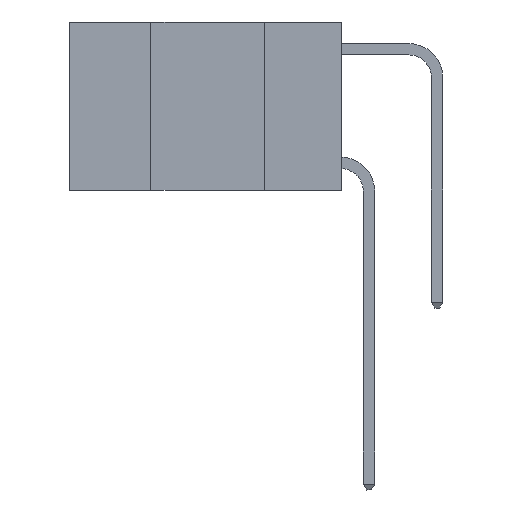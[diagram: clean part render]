
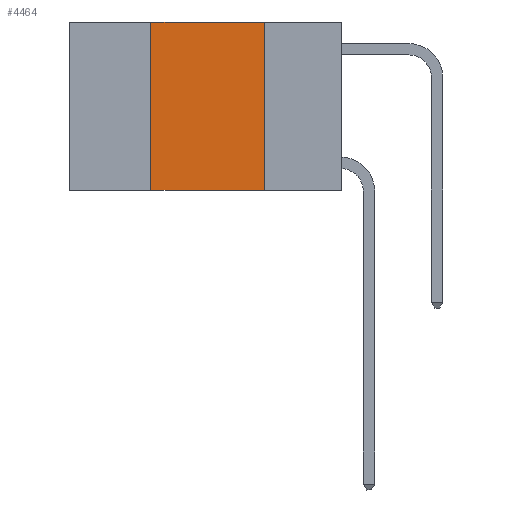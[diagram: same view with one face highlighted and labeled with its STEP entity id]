
A CAD part, left-side view. The second image highlights one B-rep face of the part: STEP entity #4464.
In plain terms, the highlighted planar face has unit normal (-1, 0, 0).
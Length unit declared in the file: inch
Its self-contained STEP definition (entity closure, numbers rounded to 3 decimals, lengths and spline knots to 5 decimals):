
#436 = DIRECTION ( 'NONE',  ( 0., 0., -1. ) ) ;
#487 = EDGE_CURVE ( 'NONE', #7042, #10571, #1868, .T. ) ;
#671 = CARTESIAN_POINT ( 'NONE',  ( 0., 0.6, 0. ) ) ;
#967 = LINE ( 'NONE', #9400, #10629 ) ;
#1220 = EDGE_CURVE ( 'NONE', #10571, #7074, #3609, .T. ) ;
#1868 = LINE ( 'NONE', #4923, #3776 ) ;
#2463 = DIRECTION ( 'NONE',  ( 0., -1., 0. ) ) ;
#2517 = ORIENTED_EDGE ( 'NONE', *, *, #3812, .T. ) ;
#2617 = CARTESIAN_POINT ( 'NONE',  ( 0., 0.42, 0. ) ) ;
#2693 = CARTESIAN_POINT ( 'NONE',  ( 0., 0.17, -0.37 ) ) ;
#3609 = LINE ( 'NONE', #4125, #8135 ) ;
#3776 = VECTOR ( 'NONE', #5828, 39.37008 ) ;
#3812 = EDGE_CURVE ( 'NONE', #9133, #7074, #7663, .T. ) ;
#3983 = DIRECTION ( 'NONE',  ( 0., 0., 1. ) ) ;
#4125 = CARTESIAN_POINT ( 'NONE',  ( 0., 0.17, 0. ) ) ;
#4393 = DIRECTION ( 'NONE',  ( 1., 0., 0. ) ) ;
#4464 = ADVANCED_FACE ( 'NONE', ( #5393 ), #9779, .F. ) ;
#4502 = ORIENTED_EDGE ( 'NONE', *, *, #11682, .F. ) ;
#4923 = CARTESIAN_POINT ( 'NONE',  ( 0., 0.6, 0. ) ) ;
#5208 = AXIS2_PLACEMENT_3D ( 'NONE', #671, #4393, #10672 ) ;
#5270 = VECTOR ( 'NONE', #2463, 39.37008 ) ;
#5393 = FACE_OUTER_BOUND ( 'NONE', #11117, .T. ) ;
#5828 = DIRECTION ( 'NONE',  ( 0., -1., 0. ) ) ;
#7042 = VERTEX_POINT ( 'NONE', #2617 ) ;
#7074 = VERTEX_POINT ( 'NONE', #2693 ) ;
#7663 = LINE ( 'NONE', #7907, #5270 ) ;
#7907 = CARTESIAN_POINT ( 'NONE',  ( 0., 0.6, -0.37 ) ) ;
#8135 = VECTOR ( 'NONE', #436, 39.37008 ) ;
#8259 = CARTESIAN_POINT ( 'NONE',  ( 0., 0.17, 0. ) ) ;
#9133 = VERTEX_POINT ( 'NONE', #11428 ) ;
#9400 = CARTESIAN_POINT ( 'NONE',  ( 0., 0.42, 0. ) ) ;
#9723 = ORIENTED_EDGE ( 'NONE', *, *, #1220, .F. ) ;
#9779 = PLANE ( 'NONE',  #5208 ) ;
#10181 = ORIENTED_EDGE ( 'NONE', *, *, #487, .F. ) ;
#10571 = VERTEX_POINT ( 'NONE', #8259 ) ;
#10629 = VECTOR ( 'NONE', #3983, 39.37008 ) ;
#10672 = DIRECTION ( 'NONE',  ( 0., 0., -1. ) ) ;
#11117 = EDGE_LOOP ( 'NONE', ( #9723, #10181, #4502, #2517 ) ) ;
#11428 = CARTESIAN_POINT ( 'NONE',  ( 0., 0.42, -0.37 ) ) ;
#11682 = EDGE_CURVE ( 'NONE', #9133, #7042, #967, .T. ) ;
